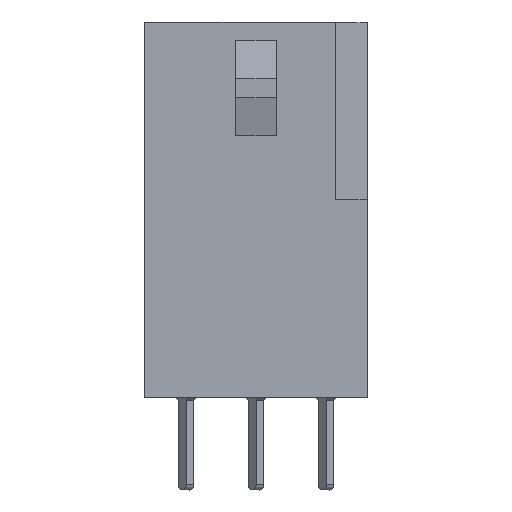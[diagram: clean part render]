
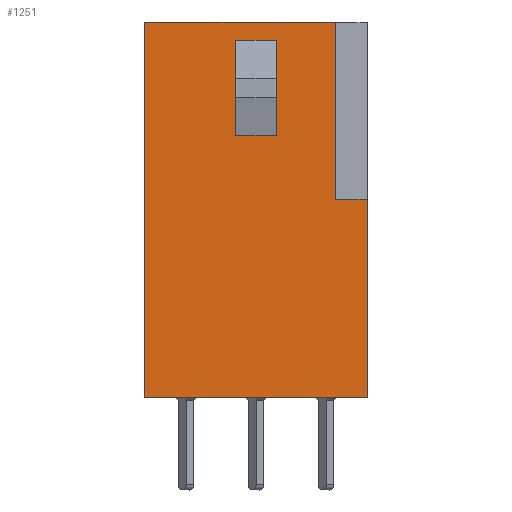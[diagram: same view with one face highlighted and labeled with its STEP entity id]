
A CAD part, top view. The second image highlights one B-rep face of the part: STEP entity #1251.
In plain terms, the highlighted planar face has unit normal (0, 0, 1).
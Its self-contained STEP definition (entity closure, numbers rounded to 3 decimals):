
#36 = VECTOR ( 'NONE', #1259, 1000. ) ;
#126 = ORIENTED_EDGE ( 'NONE', *, *, #5774, .F. ) ;
#206 = VECTOR ( 'NONE', #4113, 1000. ) ;
#227 = VERTEX_POINT ( 'NONE', #3478 ) ;
#252 = VECTOR ( 'NONE', #3049, 1000. ) ;
#323 = LINE ( 'NONE', #1889, #4264 ) ;
#394 = FACE_BOUND ( 'NONE', #2858, .T. ) ;
#414 = LINE ( 'NONE', #5050, #206 ) ;
#434 = VERTEX_POINT ( 'NONE', #5553 ) ;
#695 = VERTEX_POINT ( 'NONE', #5712 ) ;
#868 = CARTESIAN_POINT ( 'NONE',  ( 2.819, 3.608, 2.54 ) ) ;
#1066 = CARTESIAN_POINT ( 'NONE',  ( -2.324, 10.033, 2.54 ) ) ;
#1132 = EDGE_CURVE ( 'NONE', #434, #5605, #3286, .T. ) ;
#1222 = ORIENTED_EDGE ( 'NONE', *, *, #5066, .F. ) ;
#1251 = ADVANCED_FACE ( 'NONE', ( #394, #2425 ), #4606, .T. ) ;
#1252 = VECTOR ( 'NONE', #4458, 1000. ) ;
#1259 = DIRECTION ( 'NONE',  ( -1., 0., 0. ) ) ;
#1276 = LINE ( 'NONE', #1723, #36 ) ;
#1333 = CARTESIAN_POINT ( 'NONE',  ( 5.105, 8.991, 2.54 ) ) ;
#1568 = LINE ( 'NONE', #3731, #2020 ) ;
#1573 = VERTEX_POINT ( 'NONE', #4429 ) ;
#1723 = CARTESIAN_POINT ( 'NONE',  ( 7.339, 3.608, 2.54 ) ) ;
#1754 = ORIENTED_EDGE ( 'NONE', *, *, #2674, .T. ) ;
#1831 = EDGE_CURVE ( 'NONE', #1573, #4395, #323, .T. ) ;
#1889 = CARTESIAN_POINT ( 'NONE',  ( -2.324, 0., 2.54 ) ) ;
#1909 = DIRECTION ( 'NONE',  ( -1., 0., 0. ) ) ;
#2020 = VECTOR ( 'NONE', #2750, 1000. ) ;
#2133 = VECTOR ( 'NONE', #2174, 1000. ) ;
#2135 = EDGE_LOOP ( 'NONE', ( #4767, #3620, #1222, #3616, #1754, #3101 ) ) ;
#2174 = DIRECTION ( 'NONE',  ( 1., 0., 0. ) ) ;
#2196 = VERTEX_POINT ( 'NONE', #1333 ) ;
#2201 = CARTESIAN_POINT ( 'NONE',  ( -2.324, -11.176, 2.54 ) ) ;
#2236 = CARTESIAN_POINT ( 'NONE',  ( 8.445, 10.033, 2.54 ) ) ;
#2274 = CARTESIAN_POINT ( 'NONE',  ( 10.249, -11.176, 2.54 ) ) ;
#2425 = FACE_OUTER_BOUND ( 'NONE', #2135, .T. ) ;
#2579 = EDGE_CURVE ( 'NONE', #227, #2196, #414, .T. ) ;
#2626 = LINE ( 'NONE', #2274, #6088 ) ;
#2646 = VERTEX_POINT ( 'NONE', #2236 ) ;
#2650 = DIRECTION ( 'NONE',  ( 0., 0., 1. ) ) ;
#2674 = EDGE_CURVE ( 'NONE', #695, #2828, #3536, .T. ) ;
#2729 = DIRECTION ( 'NONE',  ( 1., 0., 0. ) ) ;
#2750 = DIRECTION ( 'NONE',  ( 1., 0., 0. ) ) ;
#2828 = VERTEX_POINT ( 'NONE', #4229 ) ;
#2858 = EDGE_LOOP ( 'NONE', ( #4348, #5060, #126, #5296 ) ) ;
#3049 = DIRECTION ( 'NONE',  ( 0., -1., 0. ) ) ;
#3101 = ORIENTED_EDGE ( 'NONE', *, *, #5219, .T. ) ;
#3286 = LINE ( 'NONE', #5889, #252 ) ;
#3370 = DIRECTION ( 'NONE',  ( 0., 1., 0. ) ) ;
#3437 = CARTESIAN_POINT ( 'NONE',  ( 8.445, 44.802, 2.54 ) ) ;
#3478 = CARTESIAN_POINT ( 'NONE',  ( 5.105, 3.608, 2.54 ) ) ;
#3536 = LINE ( 'NONE', #4607, #2133 ) ;
#3588 = EDGE_CURVE ( 'NONE', #695, #3760, #5454, .T. ) ;
#3616 = ORIENTED_EDGE ( 'NONE', *, *, #3588, .F. ) ;
#3620 = ORIENTED_EDGE ( 'NONE', *, *, #5968, .F. ) ;
#3709 = CARTESIAN_POINT ( 'NONE',  ( 10.249, 0., 2.54 ) ) ;
#3718 = CARTESIAN_POINT ( 'NONE',  ( 7.339, 8.991, 2.54 ) ) ;
#3726 = DIRECTION ( 'NONE',  ( 1., 0., 0. ) ) ;
#3731 = CARTESIAN_POINT ( 'NONE',  ( -2.324, 10.033, 2.54 ) ) ;
#3760 = VERTEX_POINT ( 'NONE', #1066 ) ;
#4113 = DIRECTION ( 'NONE',  ( 0., 1., 0. ) ) ;
#4128 = DIRECTION ( 'NONE',  ( 0., 1., 0. ) ) ;
#4229 = CARTESIAN_POINT ( 'NONE',  ( 10.249, -11.176, 2.54 ) ) ;
#4264 = VECTOR ( 'NONE', #3726, 1000. ) ;
#4348 = ORIENTED_EDGE ( 'NONE', *, *, #4388, .T. ) ;
#4388 = EDGE_CURVE ( 'NONE', #227, #5605, #1276, .T. ) ;
#4395 = VERTEX_POINT ( 'NONE', #3709 ) ;
#4429 = CARTESIAN_POINT ( 'NONE',  ( 8.445, 0., 2.54 ) ) ;
#4458 = DIRECTION ( 'NONE',  ( 0., -1., 0. ) ) ;
#4606 = PLANE ( 'NONE',  #5250 ) ;
#4607 = CARTESIAN_POINT ( 'NONE',  ( -2.324, -11.176, 2.54 ) ) ;
#4622 = LINE ( 'NONE', #3437, #1252 ) ;
#4767 = ORIENTED_EDGE ( 'NONE', *, *, #1831, .F. ) ;
#4830 = CARTESIAN_POINT ( 'NONE',  ( -2.324, -11.176, 2.54 ) ) ;
#5050 = CARTESIAN_POINT ( 'NONE',  ( 5.105, 8.992, 2.54 ) ) ;
#5051 = LINE ( 'NONE', #3718, #5284 ) ;
#5060 = ORIENTED_EDGE ( 'NONE', *, *, #1132, .F. ) ;
#5066 = EDGE_CURVE ( 'NONE', #3760, #2646, #1568, .T. ) ;
#5219 = EDGE_CURVE ( 'NONE', #2828, #4395, #2626, .T. ) ;
#5250 = AXIS2_PLACEMENT_3D ( 'NONE', #2201, #2650, #2729 ) ;
#5284 = VECTOR ( 'NONE', #1909, 1000. ) ;
#5296 = ORIENTED_EDGE ( 'NONE', *, *, #2579, .F. ) ;
#5454 = LINE ( 'NONE', #4830, #5522 ) ;
#5522 = VECTOR ( 'NONE', #3370, 1000. ) ;
#5553 = CARTESIAN_POINT ( 'NONE',  ( 2.819, 8.991, 2.54 ) ) ;
#5605 = VERTEX_POINT ( 'NONE', #868 ) ;
#5712 = CARTESIAN_POINT ( 'NONE',  ( -2.324, -11.176, 2.54 ) ) ;
#5774 = EDGE_CURVE ( 'NONE', #2196, #434, #5051, .T. ) ;
#5889 = CARTESIAN_POINT ( 'NONE',  ( 2.819, 8.992, 2.54 ) ) ;
#5968 = EDGE_CURVE ( 'NONE', #2646, #1573, #4622, .T. ) ;
#6088 = VECTOR ( 'NONE', #4128, 1000. ) ;
